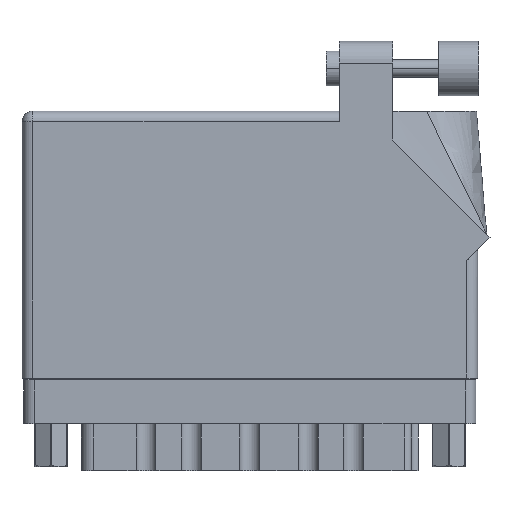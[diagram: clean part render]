
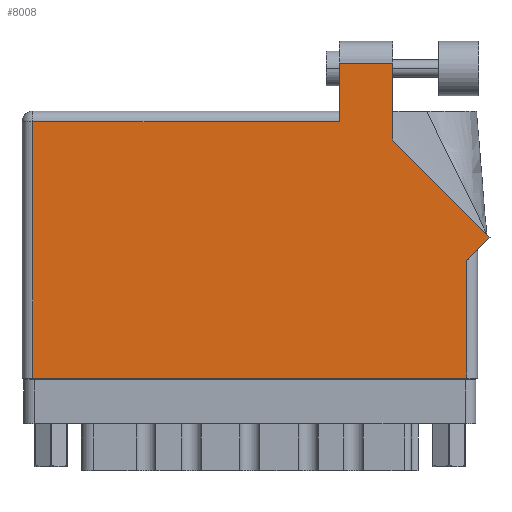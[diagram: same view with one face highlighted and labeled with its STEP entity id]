
A CAD part, front view. The second image highlights one B-rep face of the part: STEP entity #8008.
In plain terms, the highlighted face is planar.
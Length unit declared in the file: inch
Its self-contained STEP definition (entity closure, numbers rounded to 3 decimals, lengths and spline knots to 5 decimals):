
#393 = EDGE_CURVE ( 'NONE', #16459, #47211, #42526, .T. ) ;
#774 = ORIENTED_EDGE ( 'NONE', *, *, #14801, .T. ) ;
#804 = CARTESIAN_POINT ( 'NONE',  ( 0., 1.53, 0. ) ) ;
#2702 = LINE ( 'NONE', #44087, #38176 ) ;
#3265 = VERTEX_POINT ( 'NONE', #15502 ) ;
#3666 = VECTOR ( 'NONE', #32901, 39.37008 ) ;
#4709 = VECTOR ( 'NONE', #14012, 39.37008 ) ;
#6322 = VERTEX_POINT ( 'NONE', #16048 ) ;
#6846 = LINE ( 'NONE', #31418, #34056 ) ;
#7549 = CARTESIAN_POINT ( 'NONE',  ( 1.819, 1.468, 0. ) ) ;
#7687 = DIRECTION ( 'NONE',  ( 0.707, 0.707, 0. ) ) ;
#7723 = CARTESIAN_POINT ( 'NONE',  ( 2.126, 1.805, 0. ) ) ;
#8008 = ADVANCED_FACE ( 'NONE', ( #50424 ), #58868, .F. ) ;
#12234 = DIRECTION ( 'NONE',  ( -0.707, 0.707, 0. ) ) ;
#13087 = CARTESIAN_POINT ( 'NONE',  ( 0., 1.468, 0. ) ) ;
#14012 = DIRECTION ( 'NONE',  ( 0., 1., 0. ) ) ;
#14801 = EDGE_CURVE ( 'NONE', #29586, #3265, #17186, .T. ) ;
#15502 = CARTESIAN_POINT ( 'NONE',  ( 2.55, 0., 0. ) ) ;
#16048 = CARTESIAN_POINT ( 'NONE',  ( 2.68271, 0.80771, 0. ) ) ;
#16459 = VERTEX_POINT ( 'NONE', #7549 ) ;
#16480 = LINE ( 'NONE', #56817, #3666 ) ;
#17186 = LINE ( 'NONE', #31794, #43603 ) ;
#17262 = CARTESIAN_POINT ( 'NONE',  ( 0.062, 0., 0. ) ) ;
#17672 = VECTOR ( 'NONE', #56827, 39.37008 ) ;
#19783 = LINE ( 'NONE', #33916, #55169 ) ;
#20455 = EDGE_CURVE ( 'NONE', #57925, #6322, #36863, .T. ) ;
#22352 = VERTEX_POINT ( 'NONE', #32947 ) ;
#23382 = CARTESIAN_POINT ( 'NONE',  ( 2.55, 0.675, 0. ) ) ;
#24317 = EDGE_CURVE ( 'NONE', #3265, #57925, #19783, .T. ) ;
#25414 = AXIS2_PLACEMENT_3D ( 'NONE', #804, #53836, #44622 ) ;
#26721 = ORIENTED_EDGE ( 'NONE', *, *, #27495, .T. ) ;
#27495 = EDGE_CURVE ( 'NONE', #57814, #16459, #2702, .T. ) ;
#29165 = CARTESIAN_POINT ( 'NONE',  ( 2.126, 1.36442, 0. ) ) ;
#29586 = VERTEX_POINT ( 'NONE', #30314 ) ;
#30314 = CARTESIAN_POINT ( 'NONE',  ( 0.062, 0., 0. ) ) ;
#31418 = CARTESIAN_POINT ( 'NONE',  ( 2.68271, 0.80771, 0. ) ) ;
#31794 = CARTESIAN_POINT ( 'NONE',  ( 0., 0., 0. ) ) ;
#32901 = DIRECTION ( 'NONE',  ( -1., 0., 0. ) ) ;
#32947 = CARTESIAN_POINT ( 'NONE',  ( 2.126, 1.36442, 0. ) ) ;
#33916 = CARTESIAN_POINT ( 'NONE',  ( 2.55, 0.737, 0. ) ) ;
#34056 = VECTOR ( 'NONE', #12234, 39.37008 ) ;
#36599 = CARTESIAN_POINT ( 'NONE',  ( 2.612, 0.737, 0. ) ) ;
#36863 = LINE ( 'NONE', #36599, #40572 ) ;
#38176 = VECTOR ( 'NONE', #49519, 39.37008 ) ;
#38979 = DIRECTION ( 'NONE',  ( 0., 1., 0. ) ) ;
#39425 = LINE ( 'NONE', #29165, #4709 ) ;
#40572 = VECTOR ( 'NONE', #7687, 39.37008 ) ;
#41279 = EDGE_CURVE ( 'NONE', #6322, #22352, #6846, .T. ) ;
#42090 = CARTESIAN_POINT ( 'NONE',  ( 1.819, 1.805, 0. ) ) ;
#42453 = ORIENTED_EDGE ( 'NONE', *, *, #20455, .T. ) ;
#42526 = LINE ( 'NONE', #13087, #17672 ) ;
#43185 = ORIENTED_EDGE ( 'NONE', *, *, #43640, .T. ) ;
#43603 = VECTOR ( 'NONE', #46296, 39.37008 ) ;
#43640 = EDGE_CURVE ( 'NONE', #47211, #29586, #61303, .T. ) ;
#43750 = ORIENTED_EDGE ( 'NONE', *, *, #393, .T. ) ;
#44087 = CARTESIAN_POINT ( 'NONE',  ( 1.819, 1.53, 0. ) ) ;
#44622 = DIRECTION ( 'NONE',  ( -1., 0., 0. ) ) ;
#46296 = DIRECTION ( 'NONE',  ( 1., 0., 0. ) ) ;
#46928 = VERTEX_POINT ( 'NONE', #7723 ) ;
#47211 = VERTEX_POINT ( 'NONE', #48736 ) ;
#47271 = ORIENTED_EDGE ( 'NONE', *, *, #24317, .T. ) ;
#47781 = EDGE_CURVE ( 'NONE', #46928, #57814, #16480, .T. ) ;
#48736 = CARTESIAN_POINT ( 'NONE',  ( 0.062, 1.468, 0. ) ) ;
#49519 = DIRECTION ( 'NONE',  ( 0., -1., 0. ) ) ;
#50424 = FACE_OUTER_BOUND ( 'NONE', #54256, .T. ) ;
#50937 = DIRECTION ( 'NONE',  ( 0., -1., 0. ) ) ;
#51782 = ORIENTED_EDGE ( 'NONE', *, *, #41279, .T. ) ;
#53836 = DIRECTION ( 'NONE',  ( 0., 0., -1. ) ) ;
#54256 = EDGE_LOOP ( 'NONE', ( #57980, #57862, #26721, #43750, #43185, #774, #47271, #42453, #51782 ) ) ;
#55169 = VECTOR ( 'NONE', #38979, 39.37008 ) ;
#56794 = EDGE_CURVE ( 'NONE', #22352, #46928, #39425, .T. ) ;
#56817 = CARTESIAN_POINT ( 'NONE',  ( 1.819, 1.805, 0. ) ) ;
#56827 = DIRECTION ( 'NONE',  ( -1., 0., 0. ) ) ;
#57814 = VERTEX_POINT ( 'NONE', #42090 ) ;
#57862 = ORIENTED_EDGE ( 'NONE', *, *, #47781, .T. ) ;
#57925 = VERTEX_POINT ( 'NONE', #23382 ) ;
#57980 = ORIENTED_EDGE ( 'NONE', *, *, #56794, .T. ) ;
#58868 = PLANE ( 'NONE',  #25414 ) ;
#59798 = VECTOR ( 'NONE', #50937, 39.37008 ) ;
#61303 = LINE ( 'NONE', #17262, #59798 ) ;
